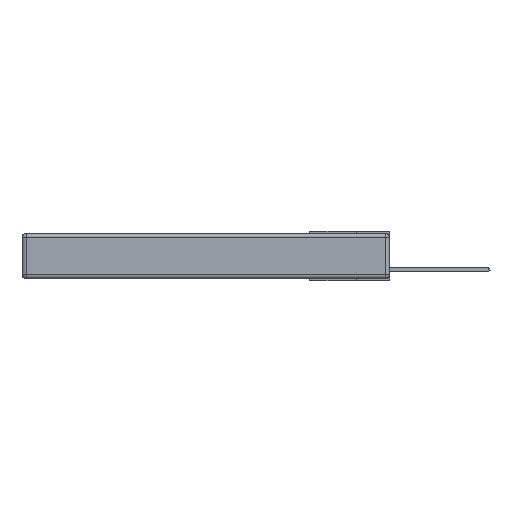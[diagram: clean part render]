
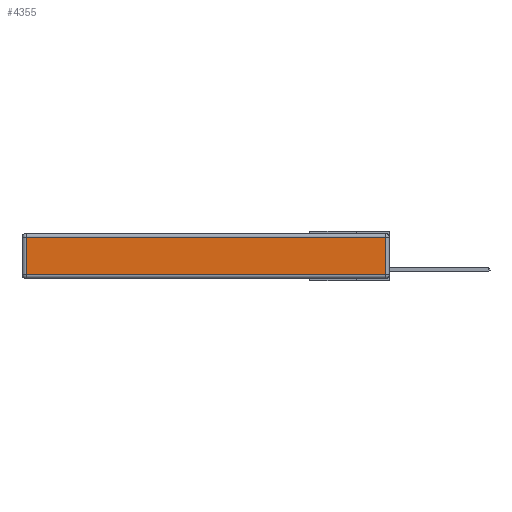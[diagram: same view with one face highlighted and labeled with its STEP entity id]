
A CAD part, left-side view. The second image highlights one B-rep face of the part: STEP entity #4355.
In plain terms, the highlighted planar face has unit normal (-1, 0, 0).
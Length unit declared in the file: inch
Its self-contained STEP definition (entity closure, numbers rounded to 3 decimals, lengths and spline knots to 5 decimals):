
#651 = VECTOR ( 'NONE', #26384, 39.37008 ) ;
#897 = LINE ( 'NONE', #12497, #16795 ) ;
#1222 = DIRECTION ( 'NONE',  ( 0., -1., 0. ) ) ;
#1814 = CARTESIAN_POINT ( 'NONE',  ( 0., 0., -0.343 ) ) ;
#4355 = ADVANCED_FACE ( 'NONE', ( #25860 ), #11269, .T. ) ;
#5076 = ORIENTED_EDGE ( 'NONE', *, *, #18326, .T. ) ;
#5094 = EDGE_CURVE ( 'NONE', #29318, #9600, #26825, .T. ) ;
#5189 = ORIENTED_EDGE ( 'NONE', *, *, #5094, .T. ) ;
#6601 = DIRECTION ( 'NONE',  ( -1., 0., 0. ) ) ;
#7806 = AXIS2_PLACEMENT_3D ( 'NONE', #1814, #6601, #9808 ) ;
#8507 = LINE ( 'NONE', #16930, #651 ) ;
#8845 = DIRECTION ( 'NONE',  ( 0., 0., -1. ) ) ;
#9600 = VERTEX_POINT ( 'NONE', #21641 ) ;
#9808 = DIRECTION ( 'NONE',  ( 0., 0., 1. ) ) ;
#11129 = VERTEX_POINT ( 'NONE', #25554 ) ;
#11269 = PLANE ( 'NONE',  #7806 ) ;
#11290 = VECTOR ( 'NONE', #8845, 39.37008 ) ;
#11298 = CARTESIAN_POINT ( 'NONE',  ( 0., 2.72, -0.343 ) ) ;
#12497 = CARTESIAN_POINT ( 'NONE',  ( 0., 0.03, -0.343 ) ) ;
#14184 = VERTEX_POINT ( 'NONE', #16724 ) ;
#15701 = CARTESIAN_POINT ( 'NONE',  ( 0., 2.72, -0.03 ) ) ;
#15718 = ORIENTED_EDGE ( 'NONE', *, *, #24042, .T. ) ;
#15882 = ORIENTED_EDGE ( 'NONE', *, *, #17701, .T. ) ;
#16724 = CARTESIAN_POINT ( 'NONE',  ( 0., 0.03, -0.313 ) ) ;
#16795 = VECTOR ( 'NONE', #29270, 39.37008 ) ;
#16930 = CARTESIAN_POINT ( 'NONE',  ( 0., 2.75, -0.03 ) ) ;
#17701 = EDGE_CURVE ( 'NONE', #14184, #11129, #897, .T. ) ;
#18182 = CARTESIAN_POINT ( 'NONE',  ( 0., 0., -0.313 ) ) ;
#18326 = EDGE_CURVE ( 'NONE', #9600, #14184, #19733, .T. ) ;
#19733 = LINE ( 'NONE', #18182, #24165 ) ;
#21641 = CARTESIAN_POINT ( 'NONE',  ( 0., 2.72, -0.313 ) ) ;
#24042 = EDGE_CURVE ( 'NONE', #11129, #29318, #8507, .T. ) ;
#24165 = VECTOR ( 'NONE', #1222, 39.37008 ) ;
#25554 = CARTESIAN_POINT ( 'NONE',  ( 0., 0.03, -0.03 ) ) ;
#25860 = FACE_OUTER_BOUND ( 'NONE', #26047, .T. ) ;
#26047 = EDGE_LOOP ( 'NONE', ( #5076, #15882, #15718, #5189 ) ) ;
#26384 = DIRECTION ( 'NONE',  ( 0., 1., 0. ) ) ;
#26825 = LINE ( 'NONE', #11298, #11290 ) ;
#29270 = DIRECTION ( 'NONE',  ( 0., 0., 1. ) ) ;
#29318 = VERTEX_POINT ( 'NONE', #15701 ) ;
